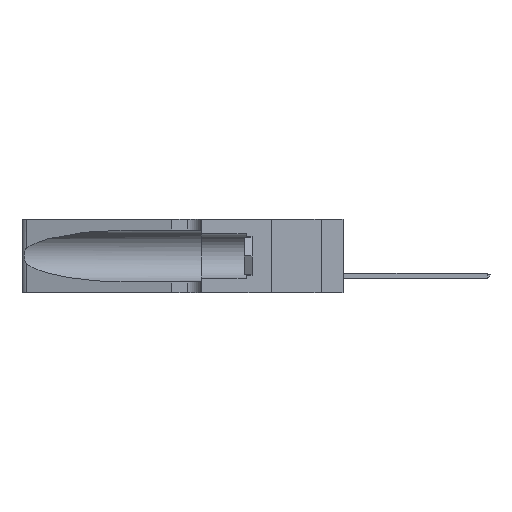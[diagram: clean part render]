
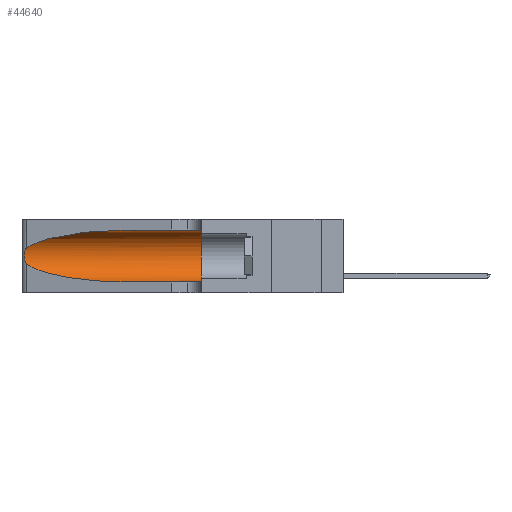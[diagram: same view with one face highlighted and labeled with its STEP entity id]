
A CAD part, left-side view. The second image highlights one B-rep face of the part: STEP entity #44640.
In plain terms, the highlighted cylindrical face has radius 3.308 mm (diameter 6.617 mm), a partial arc.
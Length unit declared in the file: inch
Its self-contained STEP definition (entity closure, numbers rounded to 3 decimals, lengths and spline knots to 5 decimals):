
#2289 = CARTESIAN_POINT ( 'NONE',  ( 0.1305, 1.61858, 0.31525 ) ) ;
#3233 = AXIS2_PLACEMENT_3D ( 'NONE', #10928, #17302, #31186 ) ;
#3261 = CIRCLE ( 'NONE', #29913, 0.13025 ) ;
#3652 = CARTESIAN_POINT ( 'NONE',  ( 0.25487, 1.22718, 0.22369 ) ) ;
#4376 = CARTESIAN_POINT ( 'NONE',  ( 0.1305, 0.35, 0.05475 ) ) ;
#6314 = CARTESIAN_POINT ( 'NONE',  ( 0.1305, 0.72297, 0.05475 ) ) ;
#6473 = CARTESIAN_POINT ( 'NONE',  ( 0.25787, 1.23484, 0.2124 ) ) ;
#7043 = CARTESIAN_POINT ( 'NONE',  ( 0.2373, 1.15595, 0.28018 ) ) ;
#7233 = EDGE_CURVE ( 'NONE', #11618, #40771, #11731, .T. ) ;
#7399 = VERTEX_POINT ( 'NONE', #21950 ) ;
#7459 = ORIENTED_EDGE ( 'NONE', *, *, #26086, .F. ) ;
#9012 = VECTOR ( 'NONE', #23771, 39.37008 ) ;
#9955 = CARTESIAN_POINT ( 'NONE',  ( 0.26075, 1.23896, 0.19203 ) ) ;
#10108 = CARTESIAN_POINT ( 'NONE',  ( 0.25639, 1.23186, 0.15144 ) ) ;
#10928 = CARTESIAN_POINT ( 'NONE',  ( 0.1305, 1.61858, 0.185 ) ) ;
#11618 = VERTEX_POINT ( 'NONE', #18593 ) ;
#11731 = LINE ( 'NONE', #40977, #9012 ) ;
#12185 = EDGE_LOOP ( 'NONE', ( #37727, #40723, #27358, #36437, #13002, #7459 ) ) ;
#12616 = DIRECTION ( 'NONE',  ( 0., -1., 0. ) ) ;
#13002 = ORIENTED_EDGE ( 'NONE', *, *, #28950, .F. ) ;
#13283 = CARTESIAN_POINT ( 'NONE',  ( 0.25487, 1.22718, 0.22369 ) ) ;
#13284 = CARTESIAN_POINT ( 'NONE',  ( 0.26018, 1.23835, 0.19895 ) ) ;
#13312 = CYLINDRICAL_SURFACE ( 'NONE', #3233, 0.13025 ) ;
#13569 = CARTESIAN_POINT ( 'NONE',  ( 0.26075, 1.23896, 0.178 ) ) ;
#14620 = EDGE_CURVE ( 'NONE', #7399, #26898, #38438, .T. ) ;
#16231 = CARTESIAN_POINT ( 'NONE',  ( 0.1305, 0.35, 0.31525 ) ) ;
#17068 = CARTESIAN_POINT ( 'NONE',  ( 0.25856, 1.23593, 0.16098 ) ) ;
#17302 = DIRECTION ( 'NONE',  ( 0., -1., 0. ) ) ;
#17707 =( BOUNDED_CURVE ( )  B_SPLINE_CURVE ( 3, ( #44427, #37609, #19800, #6314 ),
 .UNSPECIFIED., .F., .F. ) 
 B_SPLINE_CURVE_WITH_KNOTS ( ( 4, 4 ),
 ( 3.44316, 4.71239 ),
 .UNSPECIFIED. ) 
 CURVE ( )  GEOMETRIC_REPRESENTATION_ITEM ( )  RATIONAL_B_SPLINE_CURVE ( ( 1., 0.87, 0.87, 1. ) ) 
 REPRESENTATION_ITEM ( '' )  );
#18593 = CARTESIAN_POINT ( 'NONE',  ( 0.1305, 0.72297, 0.05475 ) ) ;
#19238 = LINE ( 'NONE', #2289, #34851 ) ;
#19647 = B_SPLINE_CURVE_WITH_KNOTS ( 'NONE', 3,
 ( #3652, #23900, #33983, #6473, #40659, #13284, #9955, #13569, #44141, #17068, #30821, #10108, #34277, #37767 ),
 .UNSPECIFIED., .F., .F.,
 ( 4, 2, 2, 2, 2, 2, 4 ),
 ( 0., 0.00027, 0.00053, 0.00107, 0.0016, 0.00187, 0.00214 ),
 .UNSPECIFIED. ) ;
#19800 = CARTESIAN_POINT ( 'NONE',  ( 0.18966, 0.96281, 0.05475 ) ) ;
#19834 = CARTESIAN_POINT ( 'NONE',  ( 0.1305, 0.72297, 0.31525 ) ) ;
#21092 = DIRECTION ( 'NONE',  ( 0., 1., 0. ) ) ;
#21950 = CARTESIAN_POINT ( 'NONE',  ( 0.1305, 0.72297, 0.31525 ) ) ;
#23771 = DIRECTION ( 'NONE',  ( 0., -1., 0. ) ) ;
#23900 = CARTESIAN_POINT ( 'NONE',  ( 0.25555, 1.22994, 0.2215 ) ) ;
#26086 = EDGE_CURVE ( 'NONE', #7399, #42277, #19238, .T. ) ;
#26898 = VERTEX_POINT ( 'NONE', #13283 ) ;
#27358 = ORIENTED_EDGE ( 'NONE', *, *, #31056, .T. ) ;
#27581 = EDGE_CURVE ( 'NONE', #26898, #43503, #19647, .T. ) ;
#28950 = EDGE_CURVE ( 'NONE', #42277, #40771, #3261, .T. ) ;
#29913 = AXIS2_PLACEMENT_3D ( 'NONE', #38777, #21092, #31682 ) ;
#30821 = CARTESIAN_POINT ( 'NONE',  ( 0.25789, 1.23486, 0.15765 ) ) ;
#31056 = EDGE_CURVE ( 'NONE', #43503, #11618, #17707, .T. ) ;
#31186 = DIRECTION ( 'NONE',  ( 0., 0., -1. ) ) ;
#31511 = CARTESIAN_POINT ( 'NONE',  ( 0.25487, 1.22718, 0.22369 ) ) ;
#31682 = DIRECTION ( 'NONE',  ( 0., 0., 1. ) ) ;
#33790 = CARTESIAN_POINT ( 'NONE',  ( 0.25487, 1.22718, 0.14631 ) ) ;
#33983 = CARTESIAN_POINT ( 'NONE',  ( 0.25639, 1.23184, 0.21858 ) ) ;
#34277 = CARTESIAN_POINT ( 'NONE',  ( 0.25555, 1.22993, 0.14849 ) ) ;
#34388 = FACE_OUTER_BOUND ( 'NONE', #12185, .T. ) ;
#34851 = VECTOR ( 'NONE', #12616, 39.37008 ) ;
#36437 = ORIENTED_EDGE ( 'NONE', *, *, #7233, .T. ) ;
#37609 = CARTESIAN_POINT ( 'NONE',  ( 0.2373, 1.15595, 0.08982 ) ) ;
#37727 = ORIENTED_EDGE ( 'NONE', *, *, #14620, .T. ) ;
#37767 = CARTESIAN_POINT ( 'NONE',  ( 0.25487, 1.22718, 0.14631 ) ) ;
#38438 =( BOUNDED_CURVE ( )  B_SPLINE_CURVE ( 3, ( #19834, #40082, #7043, #31511 ),
 .UNSPECIFIED., .F., .T. ) 
 B_SPLINE_CURVE_WITH_KNOTS ( ( 4, 4 ),
 ( 1.5708, 2.84003 ),
 .UNSPECIFIED. ) 
 CURVE ( )  GEOMETRIC_REPRESENTATION_ITEM ( )  RATIONAL_B_SPLINE_CURVE ( ( 1., 0.87, 0.87, 1. ) ) 
 REPRESENTATION_ITEM ( '' )  );
#38777 = CARTESIAN_POINT ( 'NONE',  ( 0.1305, 0.35, 0.185 ) ) ;
#40082 = CARTESIAN_POINT ( 'NONE',  ( 0.18966, 0.96281, 0.31525 ) ) ;
#40659 = CARTESIAN_POINT ( 'NONE',  ( 0.25854, 1.2359, 0.20912 ) ) ;
#40723 = ORIENTED_EDGE ( 'NONE', *, *, #27581, .T. ) ;
#40771 = VERTEX_POINT ( 'NONE', #4376 ) ;
#40977 = CARTESIAN_POINT ( 'NONE',  ( 0.1305, 1.61858, 0.05475 ) ) ;
#42277 = VERTEX_POINT ( 'NONE', #16231 ) ;
#43503 = VERTEX_POINT ( 'NONE', #33790 ) ;
#44141 = CARTESIAN_POINT ( 'NONE',  ( 0.26017, 1.23833, 0.17102 ) ) ;
#44427 = CARTESIAN_POINT ( 'NONE',  ( 0.25487, 1.22718, 0.14631 ) ) ;
#44640 = ADVANCED_FACE ( 'NONE', ( #34388 ), #13312, .F. ) ;
